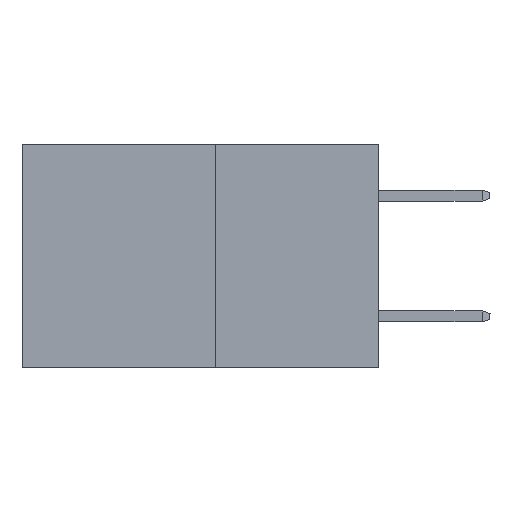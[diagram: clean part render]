
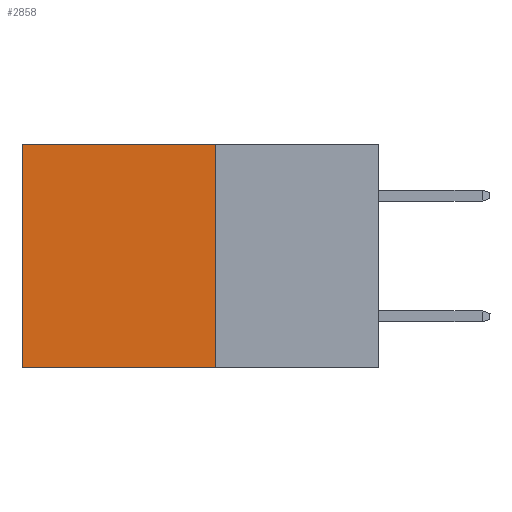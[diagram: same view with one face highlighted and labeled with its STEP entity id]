
A CAD part, left-side view. The second image highlights one B-rep face of the part: STEP entity #2858.
In plain terms, the highlighted planar face has unit normal (-1, 0, 0).
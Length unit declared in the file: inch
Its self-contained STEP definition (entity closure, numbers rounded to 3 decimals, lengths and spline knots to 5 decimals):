
#291 = CARTESIAN_POINT ( 'NONE',  ( 0.277, 0.27, 0. ) ) ;
#446 = DIRECTION ( 'NONE',  ( 0., 1., 0. ) ) ;
#572 = CARTESIAN_POINT ( 'NONE',  ( 0.277, 0.59, 0. ) ) ;
#885 = ORIENTED_EDGE ( 'NONE', *, *, #2322, .F. ) ;
#1444 = EDGE_CURVE ( 'NONE', #4280, #5231, #3988, .T. ) ;
#1461 = DIRECTION ( 'NONE',  ( 0., 1., 0. ) ) ;
#1806 = CARTESIAN_POINT ( 'NONE',  ( 0.277, 0.27, 0. ) ) ;
#1879 = DIRECTION ( 'NONE',  ( 0., 0., -1. ) ) ;
#1998 = LINE ( 'NONE', #6334, #7921 ) ;
#2169 = EDGE_CURVE ( 'NONE', #4718, #5231, #1998, .T. ) ;
#2304 = ORIENTED_EDGE ( 'NONE', *, *, #3441, .T. ) ;
#2322 = EDGE_CURVE ( 'NONE', #7293, #4718, #4049, .T. ) ;
#2858 = ADVANCED_FACE ( 'NONE', ( #6669 ), #4980, .F. ) ;
#3178 = CARTESIAN_POINT ( 'NONE',  ( 0.277, 0.59, -0.37 ) ) ;
#3242 = VECTOR ( 'NONE', #1461, 39.37008 ) ;
#3441 = EDGE_CURVE ( 'NONE', #7293, #4280, #5272, .T. ) ;
#3906 = ORIENTED_EDGE ( 'NONE', *, *, #1444, .T. ) ;
#3988 = LINE ( 'NONE', #3178, #6730 ) ;
#4049 = LINE ( 'NONE', #4202, #7913 ) ;
#4202 = CARTESIAN_POINT ( 'NONE',  ( 0.277, 0.27, -0.37 ) ) ;
#4278 = DIRECTION ( 'NONE',  ( 0., 0., -1. ) ) ;
#4280 = VERTEX_POINT ( 'NONE', #572 ) ;
#4437 = CARTESIAN_POINT ( 'NONE',  ( 0.277, 0.27, -0.37 ) ) ;
#4478 = EDGE_LOOP ( 'NONE', ( #3906, #4658, #885, #2304 ) ) ;
#4658 = ORIENTED_EDGE ( 'NONE', *, *, #2169, .F. ) ;
#4718 = VERTEX_POINT ( 'NONE', #4437 ) ;
#4980 = PLANE ( 'NONE',  #5330 ) ;
#5231 = VERTEX_POINT ( 'NONE', #7666 ) ;
#5272 = LINE ( 'NONE', #1806, #3242 ) ;
#5330 = AXIS2_PLACEMENT_3D ( 'NONE', #5500, #5488, #5410 ) ;
#5410 = DIRECTION ( 'NONE',  ( 0., 0., -1. ) ) ;
#5488 = DIRECTION ( 'NONE',  ( 1., 0., 0. ) ) ;
#5500 = CARTESIAN_POINT ( 'NONE',  ( 0.277, 0.27, -0.37 ) ) ;
#6334 = CARTESIAN_POINT ( 'NONE',  ( 0.277, 0.27, -0.37 ) ) ;
#6669 = FACE_OUTER_BOUND ( 'NONE', #4478, .T. ) ;
#6730 = VECTOR ( 'NONE', #1879, 39.37008 ) ;
#7293 = VERTEX_POINT ( 'NONE', #291 ) ;
#7666 = CARTESIAN_POINT ( 'NONE',  ( 0.277, 0.59, -0.37 ) ) ;
#7913 = VECTOR ( 'NONE', #4278, 39.37008 ) ;
#7921 = VECTOR ( 'NONE', #446, 39.37008 ) ;
